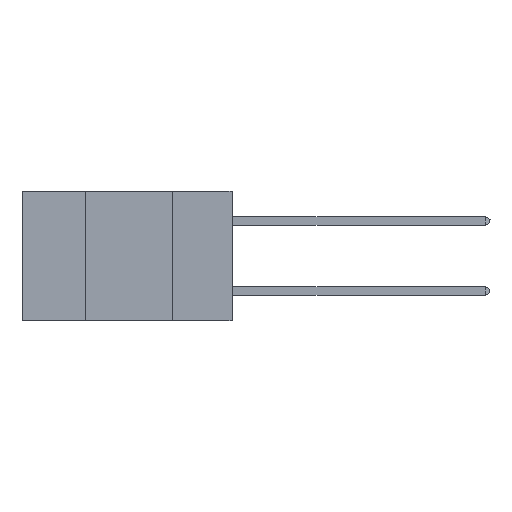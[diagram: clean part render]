
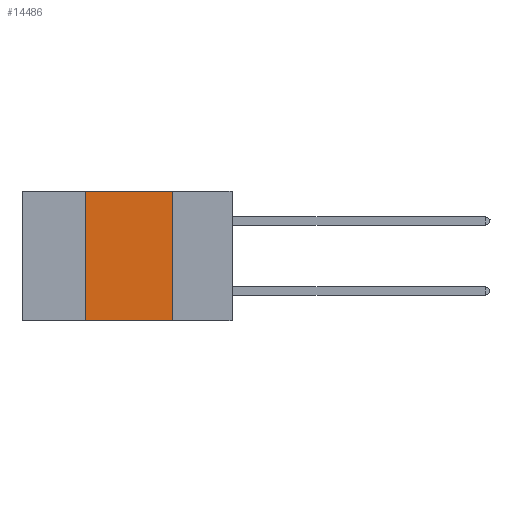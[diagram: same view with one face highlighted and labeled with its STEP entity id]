
A CAD part, left-side view. The second image highlights one B-rep face of the part: STEP entity #14486.
In plain terms, the highlighted planar face has unit normal (-1, 0, 0).
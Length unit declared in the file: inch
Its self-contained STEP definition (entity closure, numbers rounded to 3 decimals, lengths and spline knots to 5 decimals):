
#111 = EDGE_CURVE ( 'NONE', #14067, #8769, #1221, .T. ) ;
#384 = CARTESIAN_POINT ( 'NONE',  ( 0., 0.17, 0. ) ) ;
#498 = CARTESIAN_POINT ( 'NONE',  ( 0., 0.17, 0. ) ) ;
#1139 = FACE_OUTER_BOUND ( 'NONE', #4990, .T. ) ;
#1221 = LINE ( 'NONE', #12738, #10151 ) ;
#1295 = DIRECTION ( 'NONE',  ( 0., -1., 0. ) ) ;
#1481 = ORIENTED_EDGE ( 'NONE', *, *, #111, .F. ) ;
#2313 = ORIENTED_EDGE ( 'NONE', *, *, #9229, .T. ) ;
#2677 = LINE ( 'NONE', #498, #12224 ) ;
#3355 = EDGE_CURVE ( 'NONE', #3390, #14067, #8087, .T. ) ;
#3390 = VERTEX_POINT ( 'NONE', #5431 ) ;
#4082 = CARTESIAN_POINT ( 'NONE',  ( 0., 0.42, 0. ) ) ;
#4218 = EDGE_CURVE ( 'NONE', #8769, #10013, #2677, .T. ) ;
#4315 = VECTOR ( 'NONE', #1295, 39.37008 ) ;
#4703 = LINE ( 'NONE', #16107, #4315 ) ;
#4990 = EDGE_LOOP ( 'NONE', ( #11144, #1481, #14725, #2313 ) ) ;
#5431 = CARTESIAN_POINT ( 'NONE',  ( 0., 0.42, -0.37 ) ) ;
#5551 = VECTOR ( 'NONE', #13897, 39.37008 ) ;
#7313 = CARTESIAN_POINT ( 'NONE',  ( 0., 0.6, 0. ) ) ;
#8060 = AXIS2_PLACEMENT_3D ( 'NONE', #7313, #15712, #8528 ) ;
#8087 = LINE ( 'NONE', #4082, #5551 ) ;
#8528 = DIRECTION ( 'NONE',  ( 0., 0., -1. ) ) ;
#8769 = VERTEX_POINT ( 'NONE', #384 ) ;
#9229 = EDGE_CURVE ( 'NONE', #3390, #10013, #4703, .T. ) ;
#9442 = DIRECTION ( 'NONE',  ( 0., 0., -1. ) ) ;
#10013 = VERTEX_POINT ( 'NONE', #15186 ) ;
#10151 = VECTOR ( 'NONE', #12801, 39.37008 ) ;
#11144 = ORIENTED_EDGE ( 'NONE', *, *, #4218, .F. ) ;
#12224 = VECTOR ( 'NONE', #9442, 39.37008 ) ;
#12738 = CARTESIAN_POINT ( 'NONE',  ( 0., 0.6, 0. ) ) ;
#12801 = DIRECTION ( 'NONE',  ( 0., -1., 0. ) ) ;
#12846 = CARTESIAN_POINT ( 'NONE',  ( 0., 0.42, 0. ) ) ;
#13298 = PLANE ( 'NONE',  #8060 ) ;
#13897 = DIRECTION ( 'NONE',  ( 0., 0., 1. ) ) ;
#14067 = VERTEX_POINT ( 'NONE', #12846 ) ;
#14486 = ADVANCED_FACE ( 'NONE', ( #1139 ), #13298, .F. ) ;
#14725 = ORIENTED_EDGE ( 'NONE', *, *, #3355, .F. ) ;
#15186 = CARTESIAN_POINT ( 'NONE',  ( 0., 0.17, -0.37 ) ) ;
#15712 = DIRECTION ( 'NONE',  ( 1., 0., 0. ) ) ;
#16107 = CARTESIAN_POINT ( 'NONE',  ( 0., 0.6, -0.37 ) ) ;
